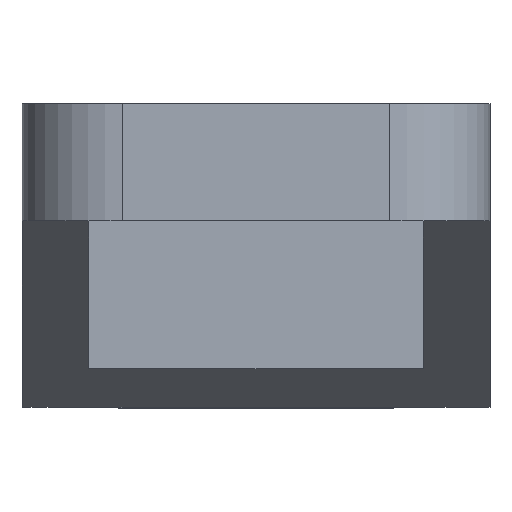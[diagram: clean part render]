
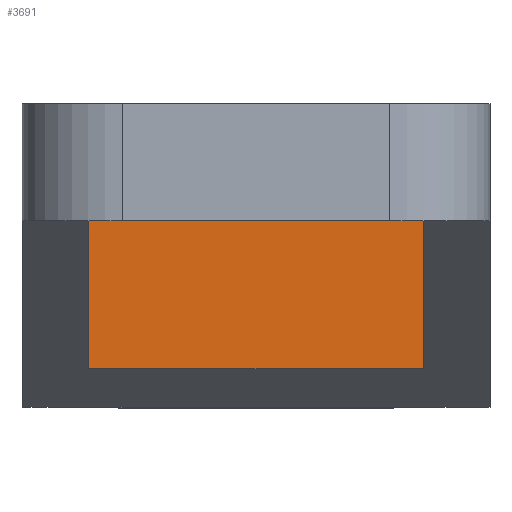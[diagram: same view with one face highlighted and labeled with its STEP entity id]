
A CAD part, front view. The second image highlights one B-rep face of the part: STEP entity #3691.
In plain terms, the highlighted planar face has unit normal (0, -1, 0).
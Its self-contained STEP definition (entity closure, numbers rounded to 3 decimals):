
#44 = PLANE('',#45);
#45 = AXIS2_PLACEMENT_3D('',#46,#47,#48);
#46 = CARTESIAN_POINT('',(-7.,-5.293,-2.401));
#47 = DIRECTION('',(0.,0.,1.));
#48 = DIRECTION('',(0.,1.,0.));
#98 = PLANE('',#99);
#99 = AXIS2_PLACEMENT_3D('',#100,#101,#102);
#100 = CARTESIAN_POINT('',(-7.,1.381,-7.972));
#101 = DIRECTION('',(0.,-0.641,-0.768));
#102 = DIRECTION('',(0.,-0.768,0.641));
#138 = VERTEX_POINT('',#139);
#139 = CARTESIAN_POINT('',(-5.,0.,-2.401));
#152 = PLANE('',#153);
#153 = AXIS2_PLACEMENT_3D('',#154,#155,#156);
#154 = CARTESIAN_POINT('',(-5.,0.,-2.4));
#155 = DIRECTION('',(-1.,0.,0.));
#156 = DIRECTION('',(0.,-1.,0.));
#163 = EDGE_CURVE('',#164,#138,#166,.T.);
#164 = VERTEX_POINT('',#165);
#165 = CARTESIAN_POINT('',(5.,0.,-2.401));
#166 = SURFACE_CURVE('',#167,(#171,#177),.PCURVE_S1.);
#167 = LINE('',#168,#169);
#168 = CARTESIAN_POINT('',(-1.,0.,-2.401));
#169 = VECTOR('',#170,1.);
#170 = DIRECTION('',(-1.,0.,0.));
#171 = PCURVE('',#44,#172);
#172 = DEFINITIONAL_REPRESENTATION('',(#173),#176);
#173 = B_SPLINE_CURVE_WITH_KNOTS('',1,(#174,#175),.UNSPECIFIED.,.F.,.F.,
  (2,2),(-7.,5.),.PIECEWISE_BEZIER_KNOTS.);
#174 = CARTESIAN_POINT('',(5.293,-13.));
#175 = CARTESIAN_POINT('',(5.293,-1.));
#176 = ( GEOMETRIC_REPRESENTATION_CONTEXT(2) 
PARAMETRIC_REPRESENTATION_CONTEXT() REPRESENTATION_CONTEXT('2D SPACE',''
  ) );
#177 = PCURVE('',#178,#183);
#178 = PLANE('',#179);
#179 = AXIS2_PLACEMENT_3D('',#180,#181,#182);
#180 = CARTESIAN_POINT('',(5.,0.,-2.4));
#181 = DIRECTION('',(0.,1.,0.));
#182 = DIRECTION('',(-1.,0.,0.));
#183 = DEFINITIONAL_REPRESENTATION('',(#184),#187);
#184 = B_SPLINE_CURVE_WITH_KNOTS('',1,(#185,#186),.UNSPECIFIED.,.F.,.F.,
  (2,2),(-7.,5.),.PIECEWISE_BEZIER_KNOTS.);
#185 = CARTESIAN_POINT('',(-1.,-0.001));
#186 = CARTESIAN_POINT('',(11.,-0.001));
#187 = ( GEOMETRIC_REPRESENTATION_CONTEXT(2) 
PARAMETRIC_REPRESENTATION_CONTEXT() REPRESENTATION_CONTEXT('2D SPACE',''
  ) );
#204 = PLANE('',#205);
#205 = AXIS2_PLACEMENT_3D('',#206,#207,#208);
#206 = CARTESIAN_POINT('',(5.,-5.778,-2.4));
#207 = DIRECTION('',(1.,0.,0.));
#208 = DIRECTION('',(0.,1.,0.));
#1856 = VERTEX_POINT('',#1857);
#1857 = CARTESIAN_POINT('',(5.,0.,-6.819));
#1876 = EDGE_CURVE('',#1877,#1856,#1879,.T.);
#1877 = VERTEX_POINT('',#1878);
#1878 = CARTESIAN_POINT('',(-5.,0.,-6.819));
#1879 = SURFACE_CURVE('',#1880,(#1884,#1890),.PCURVE_S1.);
#1880 = LINE('',#1881,#1882);
#1881 = CARTESIAN_POINT('',(-1.,0.,-6.819));
#1882 = VECTOR('',#1883,1.);
#1883 = DIRECTION('',(1.,0.,0.));
#1884 = PCURVE('',#98,#1885);
#1885 = DEFINITIONAL_REPRESENTATION('',(#1886),#1889);
#1886 = B_SPLINE_CURVE_WITH_KNOTS('',1,(#1887,#1888),.UNSPECIFIED.,.F.,
  .F.,(2,2),(-5.,7.),.PIECEWISE_BEZIER_KNOTS.);
#1887 = CARTESIAN_POINT('',(1.799,-1.));
#1888 = CARTESIAN_POINT('',(1.799,-13.));
#1889 = ( GEOMETRIC_REPRESENTATION_CONTEXT(2) 
PARAMETRIC_REPRESENTATION_CONTEXT() REPRESENTATION_CONTEXT('2D SPACE',''
  ) );
#1890 = PCURVE('',#178,#1891);
#1891 = DEFINITIONAL_REPRESENTATION('',(#1892),#1895);
#1892 = B_SPLINE_CURVE_WITH_KNOTS('',1,(#1893,#1894),.UNSPECIFIED.,.F.,
  .F.,(2,2),(-5.,7.),.PIECEWISE_BEZIER_KNOTS.);
#1893 = CARTESIAN_POINT('',(11.,-4.419));
#1894 = CARTESIAN_POINT('',(-1.,-4.419));
#1895 = ( GEOMETRIC_REPRESENTATION_CONTEXT(2) 
PARAMETRIC_REPRESENTATION_CONTEXT() REPRESENTATION_CONTEXT('2D SPACE',''
  ) );
#3669 = EDGE_CURVE('',#164,#1856,#3670,.T.);
#3670 = SURFACE_CURVE('',#3671,(#3675,#3682),.PCURVE_S1.);
#3671 = LINE('',#3672,#3673);
#3672 = CARTESIAN_POINT('',(5.,0.,-2.4));
#3673 = VECTOR('',#3674,1.);
#3674 = DIRECTION('',(0.,0.,-1.));
#3675 = PCURVE('',#204,#3676);
#3676 = DEFINITIONAL_REPRESENTATION('',(#3677),#3681);
#3677 = LINE('',#3678,#3679);
#3678 = CARTESIAN_POINT('',(5.778,0.));
#3679 = VECTOR('',#3680,1.);
#3680 = DIRECTION('',(0.,-1.));
#3681 = ( GEOMETRIC_REPRESENTATION_CONTEXT(2) 
PARAMETRIC_REPRESENTATION_CONTEXT() REPRESENTATION_CONTEXT('2D SPACE',''
  ) );
#3682 = PCURVE('',#178,#3683);
#3683 = DEFINITIONAL_REPRESENTATION('',(#3684),#3688);
#3684 = LINE('',#3685,#3686);
#3685 = CARTESIAN_POINT('',(0.,0.));
#3686 = VECTOR('',#3687,1.);
#3687 = DIRECTION('',(0.,-1.));
#3688 = ( GEOMETRIC_REPRESENTATION_CONTEXT(2) 
PARAMETRIC_REPRESENTATION_CONTEXT() REPRESENTATION_CONTEXT('2D SPACE',''
  ) );
#3691 = ADVANCED_FACE('',(#3692),#178,.F.);
#3692 = FACE_BOUND('',#3693,.F.);
#3693 = EDGE_LOOP('',(#3694,#3695,#3696,#3697));
#3694 = ORIENTED_EDGE('',*,*,#163,.F.);
#3695 = ORIENTED_EDGE('',*,*,#3669,.T.);
#3696 = ORIENTED_EDGE('',*,*,#1876,.F.);
#3697 = ORIENTED_EDGE('',*,*,#3698,.F.);
#3698 = EDGE_CURVE('',#138,#1877,#3699,.T.);
#3699 = SURFACE_CURVE('',#3700,(#3704,#3711),.PCURVE_S1.);
#3700 = LINE('',#3701,#3702);
#3701 = CARTESIAN_POINT('',(-5.,0.,-2.4));
#3702 = VECTOR('',#3703,1.);
#3703 = DIRECTION('',(0.,0.,-1.));
#3704 = PCURVE('',#178,#3705);
#3705 = DEFINITIONAL_REPRESENTATION('',(#3706),#3710);
#3706 = LINE('',#3707,#3708);
#3707 = CARTESIAN_POINT('',(10.,0.));
#3708 = VECTOR('',#3709,1.);
#3709 = DIRECTION('',(0.,-1.));
#3710 = ( GEOMETRIC_REPRESENTATION_CONTEXT(2) 
PARAMETRIC_REPRESENTATION_CONTEXT() REPRESENTATION_CONTEXT('2D SPACE',''
  ) );
#3711 = PCURVE('',#152,#3712);
#3712 = DEFINITIONAL_REPRESENTATION('',(#3713),#3717);
#3713 = LINE('',#3714,#3715);
#3714 = CARTESIAN_POINT('',(0.,0.));
#3715 = VECTOR('',#3716,1.);
#3716 = DIRECTION('',(0.,-1.));
#3717 = ( GEOMETRIC_REPRESENTATION_CONTEXT(2) 
PARAMETRIC_REPRESENTATION_CONTEXT() REPRESENTATION_CONTEXT('2D SPACE',''
  ) );
